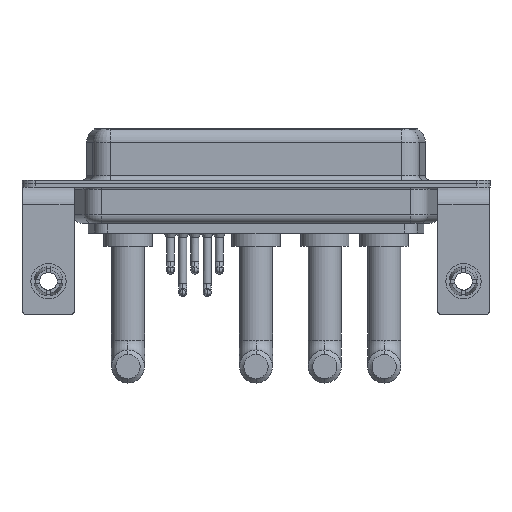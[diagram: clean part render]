
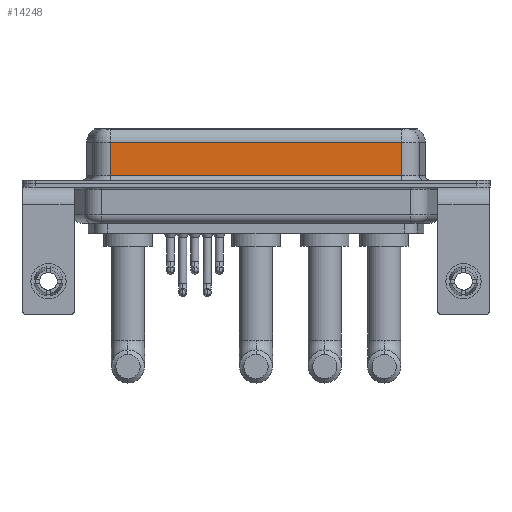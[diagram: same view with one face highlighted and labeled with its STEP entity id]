
A CAD part, front view. The second image highlights one B-rep face of the part: STEP entity #14248.
In plain terms, the highlighted planar face has unit normal (0, -1, 0).
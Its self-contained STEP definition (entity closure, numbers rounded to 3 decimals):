
#626 = CARTESIAN_POINT ( 'NONE',  ( 40.037, -3.95, 0.9 ) ) ;
#792 = LINE ( 'NONE', #19284, #6671 ) ;
#1754 = ORIENTED_EDGE ( 'NONE', *, *, #14827, .T. ) ;
#1967 = DIRECTION ( 'NONE',  ( 0., 0., 1. ) ) ;
#2681 = VECTOR ( 'NONE', #8215, 1000. ) ;
#3182 = VERTEX_POINT ( 'NONE', #8371 ) ;
#3388 = DIRECTION ( 'NONE',  ( 0., 0., -1. ) ) ;
#4659 = EDGE_LOOP ( 'NONE', ( #5813, #7406, #18643, #1754 ) ) ;
#5793 = EDGE_CURVE ( 'NONE', #3182, #15989, #11187, .T. ) ;
#5813 = ORIENTED_EDGE ( 'NONE', *, *, #19126, .F. ) ;
#6671 = VECTOR ( 'NONE', #7158, 1000. ) ;
#6712 = DIRECTION ( 'NONE',  ( 1., 0., 0. ) ) ;
#7141 = CARTESIAN_POINT ( 'NONE',  ( 7.013, -3.95, 0.9 ) ) ;
#7158 = DIRECTION ( 'NONE',  ( -1., 0., 0. ) ) ;
#7370 = VECTOR ( 'NONE', #6712, 1000. ) ;
#7406 = ORIENTED_EDGE ( 'NONE', *, *, #12417, .T. ) ;
#8215 = DIRECTION ( 'NONE',  ( 0., 0., -1. ) ) ;
#8371 = CARTESIAN_POINT ( 'NONE',  ( 7.013, -3.95, 4.65 ) ) ;
#8431 = PLANE ( 'NONE',  #19098 ) ;
#8671 = LINE ( 'NONE', #626, #7370 ) ;
#9561 = CARTESIAN_POINT ( 'NONE',  ( 40.037, -3.95, 0.9 ) ) ;
#9717 = DIRECTION ( 'NONE',  ( 0., 1., 0. ) ) ;
#11187 = LINE ( 'NONE', #15661, #2681 ) ;
#11306 = VERTEX_POINT ( 'NONE', #9561 ) ;
#11437 = VERTEX_POINT ( 'NONE', #19207 ) ;
#11580 = VECTOR ( 'NONE', #3388, 1000. ) ;
#12417 = EDGE_CURVE ( 'NONE', #11437, #3182, #792, .T. ) ;
#12785 = FACE_OUTER_BOUND ( 'NONE', #4659, .T. ) ;
#13697 = CARTESIAN_POINT ( 'NONE',  ( 40.037, -3.95, 6.4 ) ) ;
#14248 = ADVANCED_FACE ( 'NONE', ( #12785 ), #8431, .F. ) ;
#14827 = EDGE_CURVE ( 'NONE', #15989, #11306, #8671, .T. ) ;
#15198 = LINE ( 'NONE', #13697, #11580 ) ;
#15661 = CARTESIAN_POINT ( 'NONE',  ( 7.013, -3.95, 6.4 ) ) ;
#15975 = CARTESIAN_POINT ( 'NONE',  ( 40.037, -3.95, 6.4 ) ) ;
#15989 = VERTEX_POINT ( 'NONE', #7141 ) ;
#18643 = ORIENTED_EDGE ( 'NONE', *, *, #5793, .T. ) ;
#19098 = AXIS2_PLACEMENT_3D ( 'NONE', #15975, #9717, #1967 ) ;
#19126 = EDGE_CURVE ( 'NONE', #11437, #11306, #15198, .T. ) ;
#19207 = CARTESIAN_POINT ( 'NONE',  ( 40.037, -3.95, 4.65 ) ) ;
#19284 = CARTESIAN_POINT ( 'NONE',  ( 40.037, -3.95, 4.65 ) ) ;
